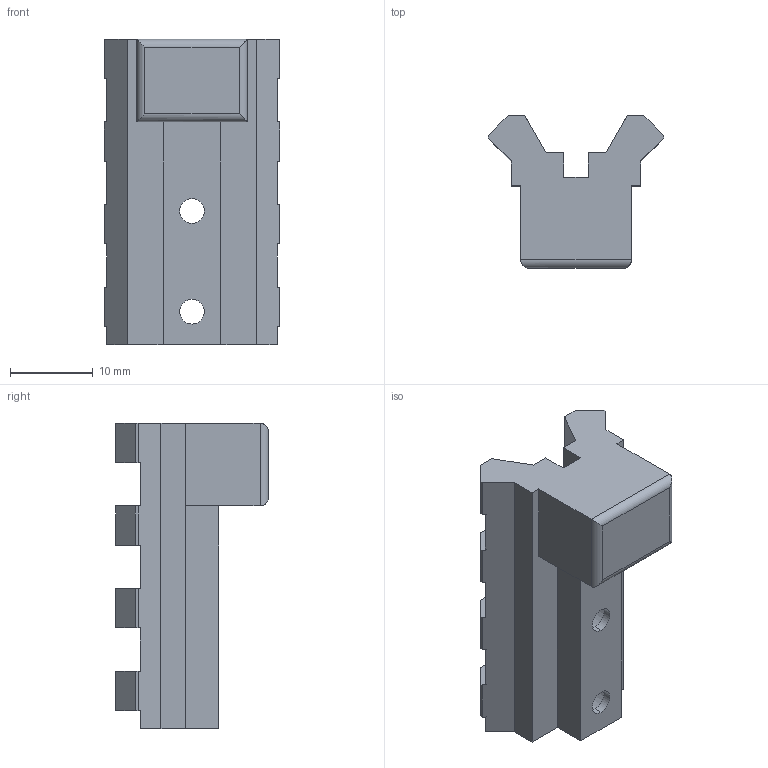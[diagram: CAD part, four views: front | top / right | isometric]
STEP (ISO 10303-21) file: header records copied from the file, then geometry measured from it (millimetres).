
FILE_DESCRIPTION (( 'STEP AP214' ), '1' );
FILE_NAME ('SightRail.STEP', '2019-11-20T13:58:43', ( '' ), ( '' ), 'SwSTEP 2.0', 'SolidWorks 2017', '' );
FILE_SCHEMA (( 'AUTOMOTIVE_DESIGN' ));
Length unit declared in the file: millimetre
Products named in the file (1): SightRail
Bounding box: 21.21 x 18.49 x 37 mm (x, y, z)
Volume: 4902 mm3; surface area: 3420.1 mm2
Topology: 1 solids, 1 shells, 88 faces, 254 edges, 168 vertices
Faces by surface type: plane 76, cylinder 12
Entity records: 2892 total; most frequent: CARTESIAN_POINT 523, ORIENTED_EDGE 508, DIRECTION 452, EDGE_CURVE 254, VECTOR 226, LINE 226, VERTEX_POINT 168, AXIS2_PLACEMENT_3D 113
